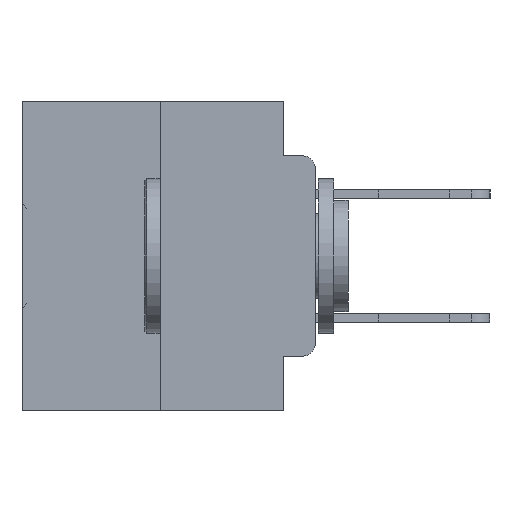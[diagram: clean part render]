
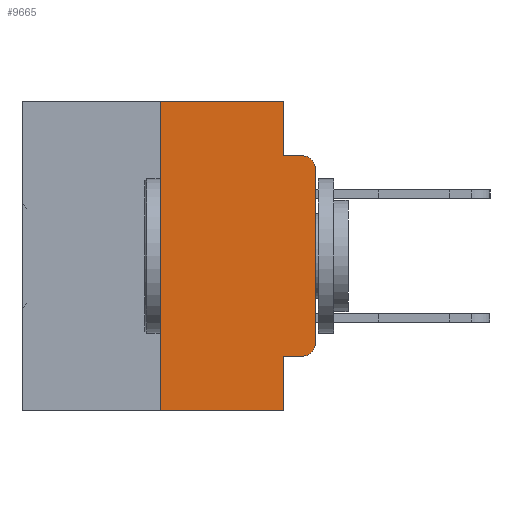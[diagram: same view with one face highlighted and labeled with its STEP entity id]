
A CAD part, left-side view. The second image highlights one B-rep face of the part: STEP entity #9665.
In plain terms, the highlighted planar face has unit normal (-1, 0, 0).
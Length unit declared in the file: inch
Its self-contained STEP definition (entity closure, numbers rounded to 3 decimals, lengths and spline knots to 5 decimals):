
#67 = DIRECTION ( 'NONE',  ( 0., -1., 0. ) ) ;
#118 = CARTESIAN_POINT ( 'NONE',  ( 0., 0., -0.1085 ) ) ;
#347 = CARTESIAN_POINT ( 'NONE',  ( 0., 0.473, 0. ) ) ;
#432 = CARTESIAN_POINT ( 'NONE',  ( 0., 0.02, -0.3915 ) ) ;
#440 = DIRECTION ( 'NONE',  ( -1., 0., 0. ) ) ;
#1044 = VECTOR ( 'NONE', #14873, 39.37008 ) ;
#2167 = VECTOR ( 'NONE', #67, 39.37008 ) ;
#2833 = EDGE_CURVE ( 'NONE', #29935, #22655, #13200, .T. ) ;
#2947 = ORIENTED_EDGE ( 'NONE', *, *, #4872, .T. ) ;
#3002 = LINE ( 'NONE', #3418, #2167 ) ;
#3028 = DIRECTION ( 'NONE',  ( 0., 0., -1. ) ) ;
#3189 = VERTEX_POINT ( 'NONE', #27865 ) ;
#3418 = CARTESIAN_POINT ( 'NONE',  ( 0., 0.051, -0.4115 ) ) ;
#4003 = CARTESIAN_POINT ( 'NONE',  ( 0., 0.051, -0.5 ) ) ;
#4259 = DIRECTION ( 'NONE',  ( 0., 0., 1. ) ) ;
#4609 = DIRECTION ( 'NONE',  ( 0., -1., 0. ) ) ;
#4872 = EDGE_CURVE ( 'NONE', #3189, #9732, #11821, .T. ) ;
#4981 = VECTOR ( 'NONE', #12688, 39.37008 ) ;
#5225 = ORIENTED_EDGE ( 'NONE', *, *, #2833, .F. ) ;
#5248 = ORIENTED_EDGE ( 'NONE', *, *, #17345, .T. ) ;
#5274 = EDGE_CURVE ( 'NONE', #22655, #14022, #12618, .T. ) ;
#5419 = VECTOR ( 'NONE', #19086, 39.37008 ) ;
#5726 = EDGE_CURVE ( 'NONE', #6116, #13835, #32785, .T. ) ;
#5809 = LINE ( 'NONE', #7439, #4981 ) ;
#5901 = CARTESIAN_POINT ( 'NONE',  ( 0., 0.051, -0.4115 ) ) ;
#6116 = VERTEX_POINT ( 'NONE', #13290 ) ;
#6818 = DIRECTION ( 'NONE',  ( 0., 0., -1. ) ) ;
#6849 = EDGE_CURVE ( 'NONE', #20037, #19114, #29406, .T. ) ;
#7261 = ORIENTED_EDGE ( 'NONE', *, *, #19188, .F. ) ;
#7439 = CARTESIAN_POINT ( 'NONE',  ( 0., 0.473, -0.5 ) ) ;
#7541 = DIRECTION ( 'NONE',  ( 0., 0., -1. ) ) ;
#7710 = AXIS2_PLACEMENT_3D ( 'NONE', #29671, #13910, #32318 ) ;
#7789 = CARTESIAN_POINT ( 'NONE',  ( 0., 0.051, 0. ) ) ;
#7931 = EDGE_CURVE ( 'NONE', #20037, #3189, #3002, .T. ) ;
#9665 = ADVANCED_FACE ( 'NONE', ( #23901 ), #29261, .F. ) ;
#9732 = VERTEX_POINT ( 'NONE', #11151 ) ;
#10383 = CARTESIAN_POINT ( 'NONE',  ( 0., 0.051, 0. ) ) ;
#11151 = CARTESIAN_POINT ( 'NONE',  ( 0., 0., -0.3915 ) ) ;
#11339 = AXIS2_PLACEMENT_3D ( 'NONE', #347, #18793, #3028 ) ;
#11787 = VECTOR ( 'NONE', #4609, 39.37008 ) ;
#11808 = LINE ( 'NONE', #19977, #31193 ) ;
#11821 = CIRCLE ( 'NONE', #26051, 0.02 ) ;
#12044 = EDGE_CURVE ( 'NONE', #9732, #14060, #28247, .T. ) ;
#12382 = ORIENTED_EDGE ( 'NONE', *, *, #5726, .F. ) ;
#12618 = LINE ( 'NONE', #27622, #11787 ) ;
#12688 = DIRECTION ( 'NONE',  ( 0., -1., 0. ) ) ;
#13133 = EDGE_CURVE ( 'NONE', #14060, #14022, #17048, .T. ) ;
#13200 = LINE ( 'NONE', #10383, #5419 ) ;
#13242 = ORIENTED_EDGE ( 'NONE', *, *, #12044, .T. ) ;
#13290 = CARTESIAN_POINT ( 'NONE',  ( 0., 0.25, -0.5 ) ) ;
#13586 = ORIENTED_EDGE ( 'NONE', *, *, #13133, .T. ) ;
#13835 = VERTEX_POINT ( 'NONE', #29632 ) ;
#13910 = DIRECTION ( 'NONE',  ( -1., 0., 0. ) ) ;
#14022 = VERTEX_POINT ( 'NONE', #21001 ) ;
#14060 = VERTEX_POINT ( 'NONE', #118 ) ;
#14873 = DIRECTION ( 'NONE',  ( 0., 0., 1. ) ) ;
#15315 = EDGE_LOOP ( 'NONE', ( #13242, #13586, #20163, #5225, #7261, #12382, #5248, #28023, #15611, #2947 ) ) ;
#15611 = ORIENTED_EDGE ( 'NONE', *, *, #7931, .T. ) ;
#17048 = CIRCLE ( 'NONE', #7710, 0.02 ) ;
#17304 = DIRECTION ( 'NONE',  ( 0., -1., 0. ) ) ;
#17345 = EDGE_CURVE ( 'NONE', #6116, #19114, #5809, .T. ) ;
#18730 = CARTESIAN_POINT ( 'NONE',  ( 0., 0.051, -0.0885 ) ) ;
#18793 = DIRECTION ( 'NONE',  ( 1., 0., 0. ) ) ;
#19086 = DIRECTION ( 'NONE',  ( 0., 0., -1. ) ) ;
#19114 = VERTEX_POINT ( 'NONE', #4003 ) ;
#19188 = EDGE_CURVE ( 'NONE', #13835, #29935, #11808, .T. ) ;
#19977 = CARTESIAN_POINT ( 'NONE',  ( 0., 0.473, 0. ) ) ;
#20037 = VERTEX_POINT ( 'NONE', #5901 ) ;
#20094 = CARTESIAN_POINT ( 'NONE',  ( 0., 0., 0. ) ) ;
#20163 = ORIENTED_EDGE ( 'NONE', *, *, #5274, .F. ) ;
#21001 = CARTESIAN_POINT ( 'NONE',  ( 0., 0.02, -0.0885 ) ) ;
#21472 = CARTESIAN_POINT ( 'NONE',  ( 0., 0.051, 0. ) ) ;
#22655 = VERTEX_POINT ( 'NONE', #18730 ) ;
#23901 = FACE_OUTER_BOUND ( 'NONE', #15315, .T. ) ;
#25778 = VECTOR ( 'NONE', #4259, 39.37008 ) ;
#26051 = AXIS2_PLACEMENT_3D ( 'NONE', #432, #440, #6818 ) ;
#27622 = CARTESIAN_POINT ( 'NONE',  ( 0., 0.051, -0.0885 ) ) ;
#27865 = CARTESIAN_POINT ( 'NONE',  ( 0., 0.02, -0.4115 ) ) ;
#28023 = ORIENTED_EDGE ( 'NONE', *, *, #6849, .F. ) ;
#28247 = LINE ( 'NONE', #20094, #1044 ) ;
#29261 = PLANE ( 'NONE',  #11339 ) ;
#29406 = LINE ( 'NONE', #7789, #33123 ) ;
#29632 = CARTESIAN_POINT ( 'NONE',  ( 0., 0.25, 0. ) ) ;
#29671 = CARTESIAN_POINT ( 'NONE',  ( 0., 0.02, -0.1085 ) ) ;
#29935 = VERTEX_POINT ( 'NONE', #21472 ) ;
#31193 = VECTOR ( 'NONE', #17304, 39.37008 ) ;
#32318 = DIRECTION ( 'NONE',  ( 0., 0., -1. ) ) ;
#32785 = LINE ( 'NONE', #33346, #25778 ) ;
#33123 = VECTOR ( 'NONE', #7541, 39.37008 ) ;
#33346 = CARTESIAN_POINT ( 'NONE',  ( 0., 0.25, 0. ) ) ;
